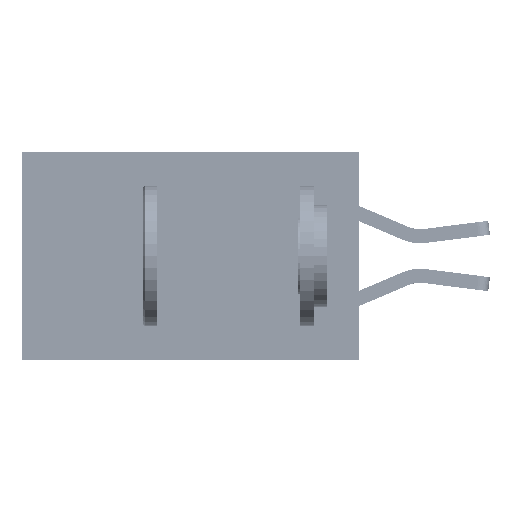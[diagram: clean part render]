
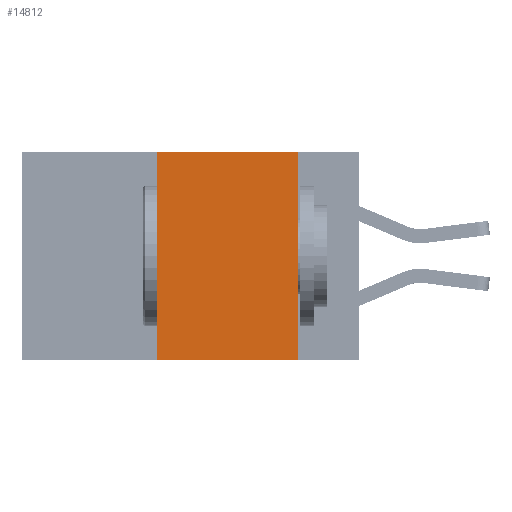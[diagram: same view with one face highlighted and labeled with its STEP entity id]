
A CAD part, left-side view. The second image highlights one B-rep face of the part: STEP entity #14812.
In plain terms, the highlighted planar face has unit normal (-1, 0, 0).
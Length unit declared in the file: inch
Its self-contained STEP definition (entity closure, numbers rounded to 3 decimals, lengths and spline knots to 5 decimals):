
#114 = VERTEX_POINT ( 'NONE', #48306 ) ;
#1227 = VERTEX_POINT ( 'NONE', #12176 ) ;
#3061 = DIRECTION ( 'NONE',  ( 0., 0., -1. ) ) ;
#4218 = VERTEX_POINT ( 'NONE', #9368 ) ;
#4728 = CARTESIAN_POINT ( 'NONE',  ( 0., 0.6, -0.37 ) ) ;
#7412 = EDGE_CURVE ( 'NONE', #4218, #1227, #16521, .T. ) ;
#9368 = CARTESIAN_POINT ( 'NONE',  ( 0., 0.11, 0. ) ) ;
#10080 = CARTESIAN_POINT ( 'NONE',  ( 0., 0.11, 0. ) ) ;
#11083 = PLANE ( 'NONE',  #13251 ) ;
#11781 = VECTOR ( 'NONE', #3061, 39.37008 ) ;
#12176 = CARTESIAN_POINT ( 'NONE',  ( 0., 0.11, -0.37 ) ) ;
#13251 = AXIS2_PLACEMENT_3D ( 'NONE', #46019, #34460, #45682 ) ;
#13850 = VECTOR ( 'NONE', #16630, 39.37008 ) ;
#14812 = ADVANCED_FACE ( 'NONE', ( #21657 ), #11083, .F. ) ;
#15884 = VECTOR ( 'NONE', #29471, 39.37008 ) ;
#16521 = LINE ( 'NONE', #10080, #11781 ) ;
#16630 = DIRECTION ( 'NONE',  ( 0., -1., 0. ) ) ;
#17509 = CARTESIAN_POINT ( 'NONE',  ( 0., 0.36, 0. ) ) ;
#21657 = FACE_OUTER_BOUND ( 'NONE', #44956, .T. ) ;
#29471 = DIRECTION ( 'NONE',  ( 0., 0., 1. ) ) ;
#30387 = ORIENTED_EDGE ( 'NONE', *, *, #48047, .F. ) ;
#30945 = CARTESIAN_POINT ( 'NONE',  ( 0., 0.36, 0. ) ) ;
#31541 = DIRECTION ( 'NONE',  ( 0., -1., 0. ) ) ;
#33826 = ORIENTED_EDGE ( 'NONE', *, *, #7412, .F. ) ;
#34460 = DIRECTION ( 'NONE',  ( 1., 0., 0. ) ) ;
#35882 = EDGE_CURVE ( 'NONE', #114, #38013, #39439, .T. ) ;
#38013 = VERTEX_POINT ( 'NONE', #30945 ) ;
#38899 = EDGE_CURVE ( 'NONE', #114, #1227, #40979, .T. ) ;
#39439 = LINE ( 'NONE', #17509, #15884 ) ;
#40203 = CARTESIAN_POINT ( 'NONE',  ( 0., 0.6, 0. ) ) ;
#40979 = LINE ( 'NONE', #4728, #42192 ) ;
#41002 = ORIENTED_EDGE ( 'NONE', *, *, #35882, .F. ) ;
#42192 = VECTOR ( 'NONE', #31541, 39.37008 ) ;
#44956 = EDGE_LOOP ( 'NONE', ( #33826, #30387, #41002, #45785 ) ) ;
#45682 = DIRECTION ( 'NONE',  ( 0., 0., -1. ) ) ;
#45733 = LINE ( 'NONE', #40203, #13850 ) ;
#45785 = ORIENTED_EDGE ( 'NONE', *, *, #38899, .T. ) ;
#46019 = CARTESIAN_POINT ( 'NONE',  ( 0., 0.6, 0. ) ) ;
#48047 = EDGE_CURVE ( 'NONE', #38013, #4218, #45733, .T. ) ;
#48306 = CARTESIAN_POINT ( 'NONE',  ( 0., 0.36, -0.37 ) ) ;
